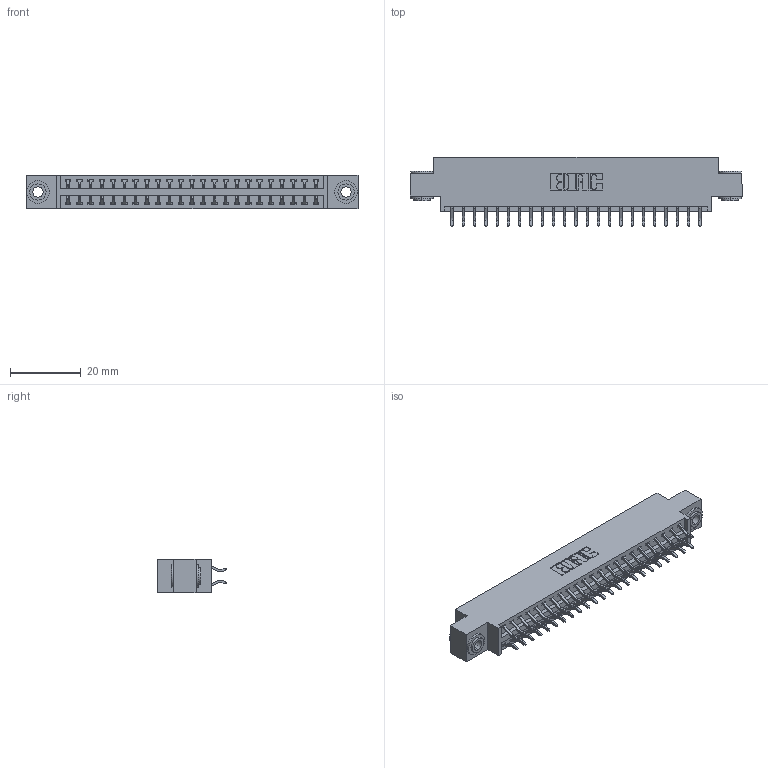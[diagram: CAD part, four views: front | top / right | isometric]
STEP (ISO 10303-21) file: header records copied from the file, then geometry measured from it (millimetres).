
FILE_DESCRIPTION (( 'STEP AP203' ), '1' );
FILE_NAME ('346-046-556-803.STEP', '2022-05-20T20:23:08', ( '' ), ( '' ), 'SwSTEP 2.0', 'SolidWorks 2020', '' );
FILE_SCHEMA (( 'CONFIG_CONTROL_DESIGN' ));
Length unit declared in the file: inch
Products named in the file (4): 345-250-002_345-250-002-102; 345-292-001_556 Tail; 346 Part_0.170 Offset - 0.156 Dia-TH; 346-046-556-803
Assembly tree (49 placements, depth 2):
  346-046-556-803
    346 Part_0.170 Offset - 0.156 Dia-TH
    345-292-001_556 Tail  x46
    345-250-002_345-250-002-102  x2
Bounding box: 93.6 x 19.57 x 9.4 mm (x, y, z)
Volume: 8824.4 mm3; surface area: 12216.7 mm2
Topology: 49 solids, 49 shells, 2846 faces, 8411 edges, 5542 vertices
Faces by surface type: plane 1898, cylinder 940, cone 8
Entity records: 18986 total; most frequent: CARTESIAN_POINT 3153, ORIENTED_EDGE 3066, DIRECTION 2847, EDGE_CURVE 1533, VECTOR 1277, LINE 1277, VERTEX_POINT 1018, AXIS2_PLACEMENT_3D 785
